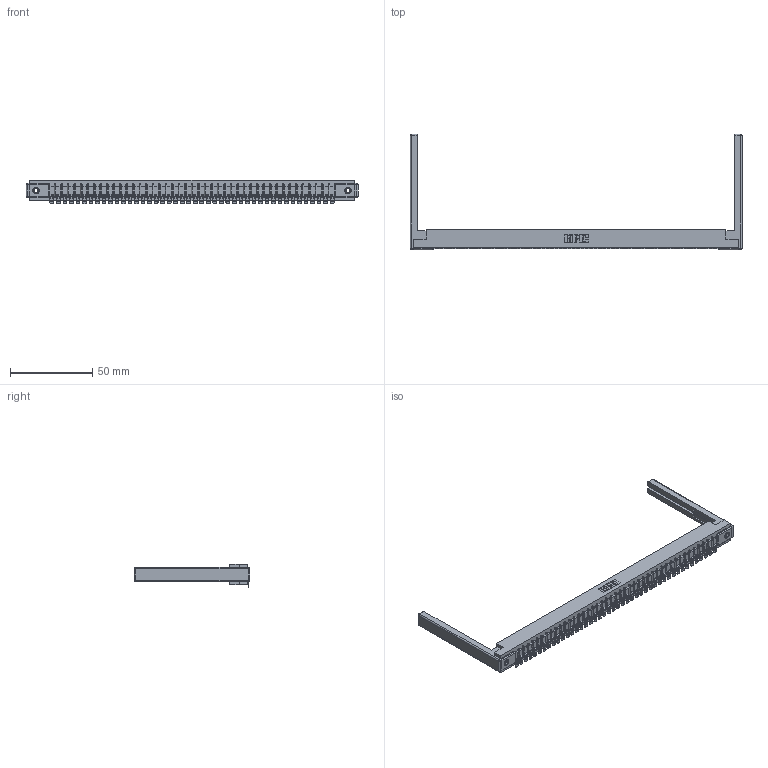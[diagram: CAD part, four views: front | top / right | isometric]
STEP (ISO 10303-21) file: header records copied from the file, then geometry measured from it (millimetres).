
FILE_DESCRIPTION (( 'STEP AP203' ), '1' );
FILE_NAME ('307-044-554-168.STEP', '2019-09-05T13:04:31', ( '' ), ( '' ), 'SwSTEP 2.0', 'SolidWorks 2016', '' );
FILE_SCHEMA (( 'CONFIG_CONTROL_DESIGN' ));
Length unit declared in the file: inch
Products named in the file (5): 307 Part_.156 Dia Mounting Holes; 345-250-001_345-250-001-102; 307-044-554-168; 307-220-068; 307-290-002_554
Assembly tree (49 placements, depth 2):
  307-044-554-168
    307 Part_.156 Dia Mounting Holes
    307-290-002_554  x44
    307-220-068  x2
    345-250-001_345-250-001-102  x2
Bounding box: 201.78 x 69.98 x 14.52 mm (x, y, z)
Volume: 26001.1 mm3; surface area: 31362.8 mm2
Topology: 49 solids, 49 shells, 3881 faces, 11845 edges, 7754 vertices
Faces by surface type: plane 2182, cylinder 1585, sphere 98, cone 12, torus 4
Entity records: 41198 total; most frequent: CARTESIAN_POINT 6915, ORIENTED_EDGE 6894, DIRECTION 6741, EDGE_CURVE 3447, LINE 2633, VECTOR 2633, VERTEX_POINT 2228, AXIS2_PLACEMENT_3D 2054
